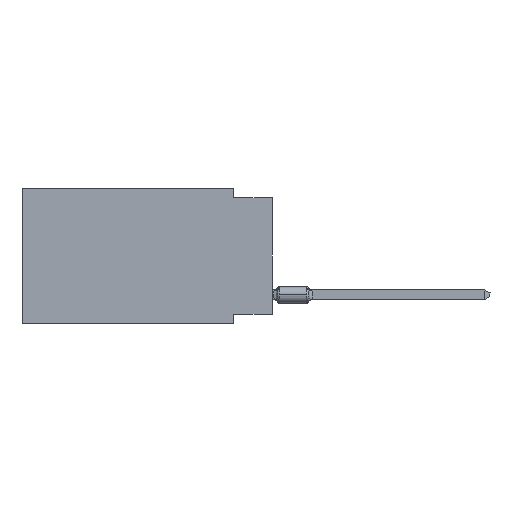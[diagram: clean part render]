
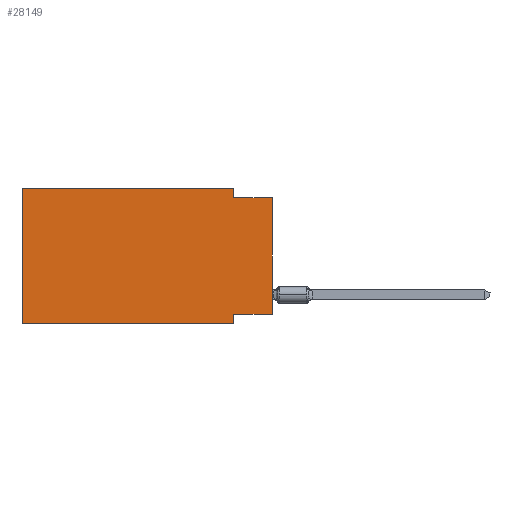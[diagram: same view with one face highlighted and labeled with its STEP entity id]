
A CAD part, left-side view. The second image highlights one B-rep face of the part: STEP entity #28149.
In plain terms, the highlighted planar face has unit normal (-1, 0, 0).
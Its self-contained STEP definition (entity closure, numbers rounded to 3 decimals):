
#1303 = EDGE_CURVE ( 'NONE', #39207, #52462, #49709, .T. ) ;
#2943 = CARTESIAN_POINT ( 'NONE',  ( 0., 0., -0.635 ) ) ;
#3743 = CARTESIAN_POINT ( 'NONE',  ( 0., 0., -8.255 ) ) ;
#3754 = LINE ( 'NONE', #49057, #24212 ) ;
#3777 = VECTOR ( 'NONE', #45184, 1000. ) ;
#6766 = ORIENTED_EDGE ( 'NONE', *, *, #31895, .F. ) ;
#11155 = CARTESIAN_POINT ( 'NONE',  ( 0., 16.383, 0. ) ) ;
#13226 = FACE_OUTER_BOUND ( 'NONE', #14413, .T. ) ;
#13816 = DIRECTION ( 'NONE',  ( 0., 0., -1. ) ) ;
#14413 = EDGE_LOOP ( 'NONE', ( #38875, #22571, #25991, #61897, #6766, #15859, #41456, #29925 ) ) ;
#15489 = DIRECTION ( 'NONE',  ( 0., 0., 1. ) ) ;
#15859 = ORIENTED_EDGE ( 'NONE', *, *, #20071, .T. ) ;
#17474 = VERTEX_POINT ( 'NONE', #34859 ) ;
#17703 = CARTESIAN_POINT ( 'NONE',  ( 0., 0., 0. ) ) ;
#18375 = CARTESIAN_POINT ( 'NONE',  ( 0., 2.54, 0. ) ) ;
#18527 = CARTESIAN_POINT ( 'NONE',  ( 0., 2.54, -8.255 ) ) ;
#19512 = DIRECTION ( 'NONE',  ( 0., 1., 0. ) ) ;
#20071 = EDGE_CURVE ( 'NONE', #58048, #44343, #45504, .T. ) ;
#20988 = CARTESIAN_POINT ( 'NONE',  ( 0., 16.383, -8.89 ) ) ;
#21304 = CARTESIAN_POINT ( 'NONE',  ( 0., 0., -0.635 ) ) ;
#21524 = AXIS2_PLACEMENT_3D ( 'NONE', #53847, #23991, #60186 ) ;
#22042 = CARTESIAN_POINT ( 'NONE',  ( 0., 16.383, -8.89 ) ) ;
#22571 = ORIENTED_EDGE ( 'NONE', *, *, #39523, .F. ) ;
#23991 = DIRECTION ( 'NONE',  ( 1., 0., 0. ) ) ;
#24212 = VECTOR ( 'NONE', #13816, 1000. ) ;
#24705 = VERTEX_POINT ( 'NONE', #18375 ) ;
#25920 = LINE ( 'NONE', #51729, #28875 ) ;
#25991 = ORIENTED_EDGE ( 'NONE', *, *, #63850, .F. ) ;
#26681 = CARTESIAN_POINT ( 'NONE',  ( 0., 16.383, 0. ) ) ;
#28141 = LINE ( 'NONE', #2943, #52659 ) ;
#28149 = ADVANCED_FACE ( 'NONE', ( #13226 ), #49464, .F. ) ;
#28875 = VECTOR ( 'NONE', #15489, 1000. ) ;
#29925 = ORIENTED_EDGE ( 'NONE', *, *, #1303, .F. ) ;
#31646 = LINE ( 'NONE', #11155, #51119 ) ;
#31698 = EDGE_CURVE ( 'NONE', #39207, #61129, #53617, .T. ) ;
#31895 = EDGE_CURVE ( 'NONE', #58048, #60405, #25920, .T. ) ;
#34859 = CARTESIAN_POINT ( 'NONE',  ( 0., 2.54, -0.635 ) ) ;
#38252 = DIRECTION ( 'NONE',  ( 0., 0., -1. ) ) ;
#38347 = VECTOR ( 'NONE', #19512, 1000. ) ;
#38875 = ORIENTED_EDGE ( 'NONE', *, *, #31698, .T. ) ;
#39207 = VERTEX_POINT ( 'NONE', #49968 ) ;
#39523 = EDGE_CURVE ( 'NONE', #17474, #61129, #28141, .T. ) ;
#40407 = EDGE_CURVE ( 'NONE', #52462, #44343, #43623, .T. ) ;
#41456 = ORIENTED_EDGE ( 'NONE', *, *, #40407, .F. ) ;
#43623 = LINE ( 'NONE', #62162, #46281 ) ;
#44161 = EDGE_CURVE ( 'NONE', #60405, #24705, #31646, .T. ) ;
#44343 = VERTEX_POINT ( 'NONE', #45030 ) ;
#45030 = CARTESIAN_POINT ( 'NONE',  ( 0., 2.54, -8.89 ) ) ;
#45184 = DIRECTION ( 'NONE',  ( 0., -1., 0. ) ) ;
#45504 = LINE ( 'NONE', #20988, #3777 ) ;
#46281 = VECTOR ( 'NONE', #38252, 1000. ) ;
#47041 = VECTOR ( 'NONE', #48251, 1000. ) ;
#48251 = DIRECTION ( 'NONE',  ( 0., 0., 1. ) ) ;
#49057 = CARTESIAN_POINT ( 'NONE',  ( 0., 2.54, 0. ) ) ;
#49464 = PLANE ( 'NONE',  #21524 ) ;
#49709 = LINE ( 'NONE', #3743, #38347 ) ;
#49968 = CARTESIAN_POINT ( 'NONE',  ( 0., 0., -8.255 ) ) ;
#51119 = VECTOR ( 'NONE', #52099, 1000. ) ;
#51729 = CARTESIAN_POINT ( 'NONE',  ( 0., 16.383, 0. ) ) ;
#52099 = DIRECTION ( 'NONE',  ( 0., -1., 0. ) ) ;
#52462 = VERTEX_POINT ( 'NONE', #18527 ) ;
#52659 = VECTOR ( 'NONE', #58979, 1000. ) ;
#53617 = LINE ( 'NONE', #17703, #47041 ) ;
#53847 = CARTESIAN_POINT ( 'NONE',  ( 0., 16.383, 0. ) ) ;
#58048 = VERTEX_POINT ( 'NONE', #22042 ) ;
#58979 = DIRECTION ( 'NONE',  ( 0., -1., 0. ) ) ;
#60186 = DIRECTION ( 'NONE',  ( 0., 0., -1. ) ) ;
#60405 = VERTEX_POINT ( 'NONE', #26681 ) ;
#61129 = VERTEX_POINT ( 'NONE', #21304 ) ;
#61897 = ORIENTED_EDGE ( 'NONE', *, *, #44161, .F. ) ;
#62162 = CARTESIAN_POINT ( 'NONE',  ( 0., 2.54, -8.89 ) ) ;
#63850 = EDGE_CURVE ( 'NONE', #24705, #17474, #3754, .T. ) ;
